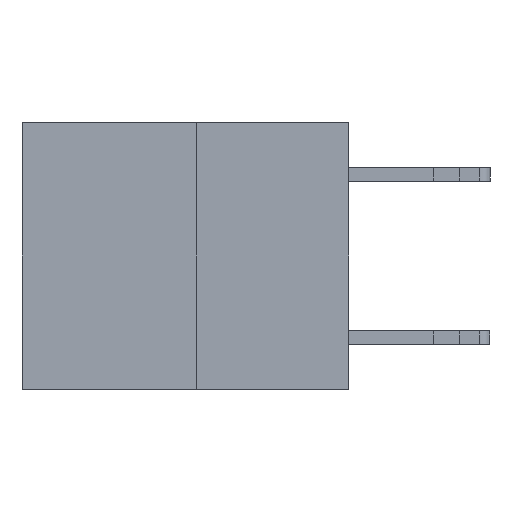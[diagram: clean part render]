
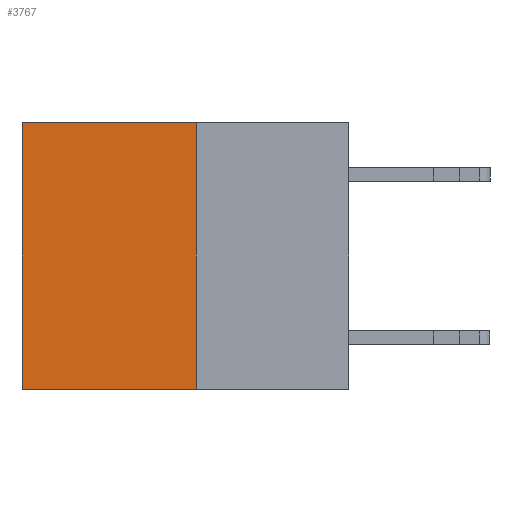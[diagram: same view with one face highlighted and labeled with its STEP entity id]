
A CAD part, left-side view. The second image highlights one B-rep face of the part: STEP entity #3767.
In plain terms, the highlighted planar face has unit normal (-1, 0, 0).
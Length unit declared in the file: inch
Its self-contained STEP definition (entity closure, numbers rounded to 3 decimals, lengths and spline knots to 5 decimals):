
#694 = DIRECTION ( 'NONE',  ( 0., 0., -1. ) ) ;
#788 = DIRECTION ( 'NONE',  ( 0., 0., -1. ) ) ;
#1068 = DIRECTION ( 'NONE',  ( 0., 1., 0. ) ) ;
#1932 = CARTESIAN_POINT ( 'NONE',  ( 0.3165, 0.28, -0.49 ) ) ;
#2042 = CARTESIAN_POINT ( 'NONE',  ( 0.3165, 0.28, 0. ) ) ;
#2636 = VERTEX_POINT ( 'NONE', #1932 ) ;
#3767 = ADVANCED_FACE ( 'NONE', ( #7103 ), #9089, .F. ) ;
#4131 = VERTEX_POINT ( 'NONE', #8501 ) ;
#4394 = CARTESIAN_POINT ( 'NONE',  ( 0.3165, 0.28, -0.49 ) ) ;
#4534 = LINE ( 'NONE', #10131, #11495 ) ;
#6390 = AXIS2_PLACEMENT_3D ( 'NONE', #9043, #6866, #7903 ) ;
#6519 = EDGE_CURVE ( 'NONE', #2636, #12980, #7533, .T. ) ;
#6825 = EDGE_CURVE ( 'NONE', #9224, #2636, #12293, .T. ) ;
#6866 = DIRECTION ( 'NONE',  ( 1., 0., 0. ) ) ;
#7103 = FACE_OUTER_BOUND ( 'NONE', #9662, .T. ) ;
#7533 = LINE ( 'NONE', #10645, #7900 ) ;
#7725 = CARTESIAN_POINT ( 'NONE',  ( 0.3165, 0.28, 0. ) ) ;
#7753 = ORIENTED_EDGE ( 'NONE', *, *, #11375, .T. ) ;
#7900 = VECTOR ( 'NONE', #1068, 39.37008 ) ;
#7903 = DIRECTION ( 'NONE',  ( 0., 0., -1. ) ) ;
#8501 = CARTESIAN_POINT ( 'NONE',  ( 0.3165, 0.6, 0. ) ) ;
#8890 = LINE ( 'NONE', #2042, #13643 ) ;
#9043 = CARTESIAN_POINT ( 'NONE',  ( 0.3165, 0.28, -0.49 ) ) ;
#9089 = PLANE ( 'NONE',  #6390 ) ;
#9224 = VERTEX_POINT ( 'NONE', #7725 ) ;
#9662 = EDGE_LOOP ( 'NONE', ( #7753, #13325, #11876, #13258 ) ) ;
#10131 = CARTESIAN_POINT ( 'NONE',  ( 0.3165, 0.6, -0.49 ) ) ;
#10645 = CARTESIAN_POINT ( 'NONE',  ( 0.3165, 0.28, -0.49 ) ) ;
#11375 = EDGE_CURVE ( 'NONE', #4131, #12980, #4534, .T. ) ;
#11495 = VECTOR ( 'NONE', #788, 39.37008 ) ;
#11539 = CARTESIAN_POINT ( 'NONE',  ( 0.3165, 0.6, -0.49 ) ) ;
#11681 = DIRECTION ( 'NONE',  ( 0., 1., 0. ) ) ;
#11733 = VECTOR ( 'NONE', #694, 39.37008 ) ;
#11876 = ORIENTED_EDGE ( 'NONE', *, *, #6825, .F. ) ;
#12293 = LINE ( 'NONE', #4394, #11733 ) ;
#12980 = VERTEX_POINT ( 'NONE', #11539 ) ;
#13258 = ORIENTED_EDGE ( 'NONE', *, *, #13378, .T. ) ;
#13325 = ORIENTED_EDGE ( 'NONE', *, *, #6519, .F. ) ;
#13378 = EDGE_CURVE ( 'NONE', #9224, #4131, #8890, .T. ) ;
#13643 = VECTOR ( 'NONE', #11681, 39.37008 ) ;
